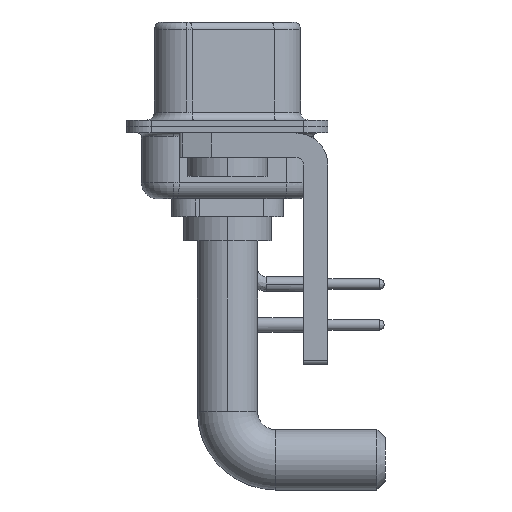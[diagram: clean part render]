
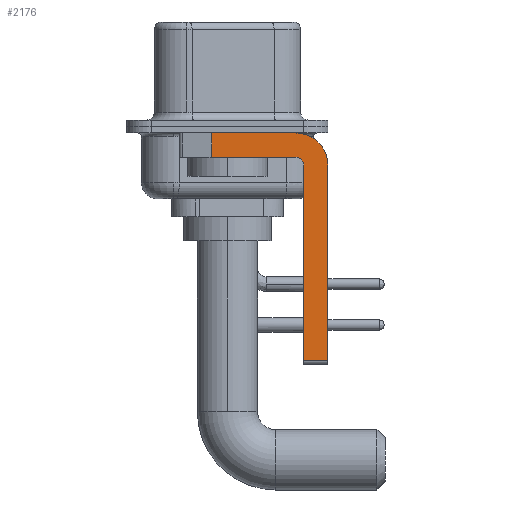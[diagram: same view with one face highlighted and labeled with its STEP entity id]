
A CAD part, left-side view. The second image highlights one B-rep face of the part: STEP entity #2176.
In plain terms, the highlighted planar face has unit normal (-1, 0, 0).
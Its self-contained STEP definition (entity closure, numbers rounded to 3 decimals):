
#251 = CARTESIAN_POINT ( 'NONE',  ( -2.9, -4.75, -14.8 ) ) ;
#755 = DIRECTION ( 'NONE',  ( 0., 0., -1. ) ) ;
#1200 = VECTOR ( 'NONE', #6182, 1000. ) ;
#1424 = LINE ( 'NONE', #27383, #16897 ) ;
#1629 = VERTEX_POINT ( 'NONE', #5476 ) ;
#2094 = ORIENTED_EDGE ( 'NONE', *, *, #21568, .F. ) ;
#2176 = ADVANCED_FACE ( 'NONE', ( #17736 ), #23772, .F. ) ;
#2449 = EDGE_CURVE ( 'NONE', #3123, #14773, #1424, .T. ) ;
#2502 = VECTOR ( 'NONE', #20003, 1000. ) ;
#3123 = VERTEX_POINT ( 'NONE', #4748 ) ;
#4080 = DIRECTION ( 'NONE',  ( 0., -1., 0. ) ) ;
#4159 = LINE ( 'NONE', #19052, #9375 ) ;
#4672 = VERTEX_POINT ( 'NONE', #21682 ) ;
#4748 = CARTESIAN_POINT ( 'NONE',  ( -2.9, -4.75, -14.55 ) ) ;
#4826 = ORIENTED_EDGE ( 'NONE', *, *, #16078, .T. ) ;
#5476 = CARTESIAN_POINT ( 'NONE',  ( -2.9, -4.75, -2.4 ) ) ;
#6182 = DIRECTION ( 'NONE',  ( 0., 0., -1. ) ) ;
#6486 = DIRECTION ( 'NONE',  ( 0., 0., 1. ) ) ;
#6568 = CARTESIAN_POINT ( 'NONE',  ( -2.9, -4.25, -2.4 ) ) ;
#6938 = AXIS2_PLACEMENT_3D ( 'NONE', #17295, #10678, #6486 ) ;
#7069 = CARTESIAN_POINT ( 'NONE',  ( -2.9, -4.25, -2.4 ) ) ;
#7176 = EDGE_CURVE ( 'NONE', #19969, #14773, #4159, .T. ) ;
#7218 = EDGE_CURVE ( 'NONE', #3123, #1629, #19471, .T. ) ;
#8358 = ORIENTED_EDGE ( 'NONE', *, *, #20359, .F. ) ;
#9375 = VECTOR ( 'NONE', #26066, 1000. ) ;
#10678 = DIRECTION ( 'NONE',  ( -1., 0., 0. ) ) ;
#11167 = CARTESIAN_POINT ( 'NONE',  ( -2.9, -6.25, -2.4 ) ) ;
#12620 = EDGE_CURVE ( 'NONE', #1629, #24122, #19042, .T. ) ;
#12619 = LINE ( 'NONE', #14879, #1200 ) ;
#13201 = ORIENTED_EDGE ( 'NONE', *, *, #12620, .F. ) ;
#13474 = DIRECTION ( 'NONE',  ( 0., -1., 0. ) ) ;
#14412 = ORIENTED_EDGE ( 'NONE', *, *, #7218, .F. ) ;
#14773 = VERTEX_POINT ( 'NONE', #16166 ) ;
#14879 = CARTESIAN_POINT ( 'NONE',  ( -2.9, 0.978, -1.9 ) ) ;
#15133 = DIRECTION ( 'NONE',  ( 1., 0., 0. ) ) ;
#15167 = ORIENTED_EDGE ( 'NONE', *, *, #7176, .F. ) ;
#15306 = LINE ( 'NONE', #15594, #18523 ) ;
#15513 = ORIENTED_EDGE ( 'NONE', *, *, #2449, .T. ) ;
#15594 = CARTESIAN_POINT ( 'NONE',  ( -2.9, 3., -0.4 ) ) ;
#15814 = DIRECTION ( 'NONE',  ( 0., 0., 1. ) ) ;
#16078 = EDGE_CURVE ( 'NONE', #19317, #4672, #12619, .T. ) ;
#16166 = CARTESIAN_POINT ( 'NONE',  ( -2.9, -6.25, -14.55 ) ) ;
#16897 = VECTOR ( 'NONE', #4080, 1000. ) ;
#16920 = AXIS2_PLACEMENT_3D ( 'NONE', #6568, #15133, #23696 ) ;
#17295 = CARTESIAN_POINT ( 'NONE',  ( -2.9, -4.25, -2.4 ) ) ;
#17736 = FACE_OUTER_BOUND ( 'NONE', #20940, .T. ) ;
#18007 = VERTEX_POINT ( 'NONE', #19240 ) ;
#18523 = VECTOR ( 'NONE', #13474, 1000. ) ;
#19042 = CIRCLE ( 'NONE', #6938, 0.5 ) ;
#19052 = CARTESIAN_POINT ( 'NONE',  ( -2.9, -6.25, -2.4 ) ) ;
#19240 = CARTESIAN_POINT ( 'NONE',  ( -2.9, -4.25, -0.4 ) ) ;
#19317 = VERTEX_POINT ( 'NONE', #21621 ) ;
#19471 = LINE ( 'NONE', #251, #21967 ) ;
#19588 = LINE ( 'NONE', #24084, #2502 ) ;
#19969 = VERTEX_POINT ( 'NONE', #11167 ) ;
#20003 = DIRECTION ( 'NONE',  ( 0., 1., 0. ) ) ;
#20359 = EDGE_CURVE ( 'NONE', #24122, #4672, #19588, .T. ) ;
#20940 = EDGE_LOOP ( 'NONE', ( #21518, #4826, #8358, #13201, #14412, #15513, #15167, #2094 ) ) ;
#21518 = ORIENTED_EDGE ( 'NONE', *, *, #27229, .F. ) ;
#21568 = EDGE_CURVE ( 'NONE', #18007, #19969, #22328, .T. ) ;
#21621 = CARTESIAN_POINT ( 'NONE',  ( -2.9, 0.978, -0.4 ) ) ;
#21682 = CARTESIAN_POINT ( 'NONE',  ( -2.9, 0.978, -1.9 ) ) ;
#21967 = VECTOR ( 'NONE', #15814, 1000. ) ;
#22328 = CIRCLE ( 'NONE', #16920, 2. ) ;
#23696 = DIRECTION ( 'NONE',  ( 0., 0., -1. ) ) ;
#23772 = PLANE ( 'NONE',  #25895 ) ;
#24084 = CARTESIAN_POINT ( 'NONE',  ( -2.9, -4.25, -1.9 ) ) ;
#24122 = VERTEX_POINT ( 'NONE', #26035 ) ;
#25895 = AXIS2_PLACEMENT_3D ( 'NONE', #7069, #26155, #755 ) ;
#26035 = CARTESIAN_POINT ( 'NONE',  ( -2.9, -4.25, -1.9 ) ) ;
#26066 = DIRECTION ( 'NONE',  ( 0., 0., -1. ) ) ;
#26155 = DIRECTION ( 'NONE',  ( 1., 0., 0. ) ) ;
#27229 = EDGE_CURVE ( 'NONE', #19317, #18007, #15306, .T. ) ;
#27383 = CARTESIAN_POINT ( 'NONE',  ( -2.9, -4.25, -14.55 ) ) ;
